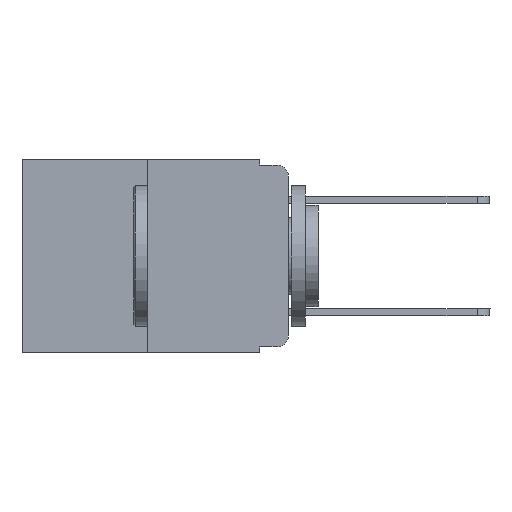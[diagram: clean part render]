
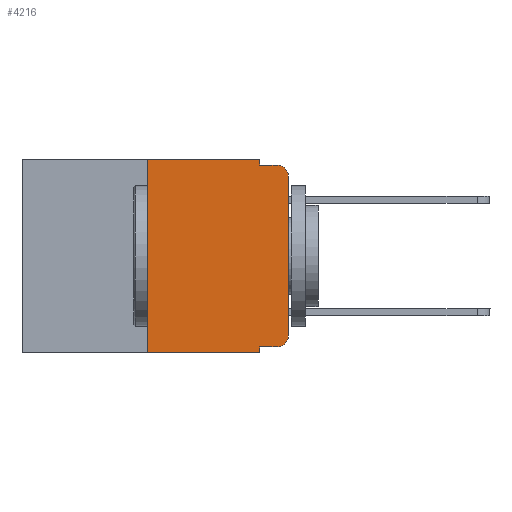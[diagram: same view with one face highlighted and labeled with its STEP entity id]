
A CAD part, left-side view. The second image highlights one B-rep face of the part: STEP entity #4216.
In plain terms, the highlighted planar face has unit normal (-1, 0, 0).
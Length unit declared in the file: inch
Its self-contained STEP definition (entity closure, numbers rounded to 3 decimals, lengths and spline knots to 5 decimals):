
#224 = ORIENTED_EDGE ( 'NONE', *, *, #13883, .T. ) ;
#556 = LINE ( 'NONE', #5082, #10669 ) ;
#725 = VECTOR ( 'NONE', #8430, 39.37008 ) ;
#908 = EDGE_CURVE ( 'NONE', #1152, #7854, #7517, .T. ) ;
#1152 = VERTEX_POINT ( 'NONE', #13057 ) ;
#1325 = DIRECTION ( 'NONE',  ( -1., 0., 0. ) ) ;
#1409 = CARTESIAN_POINT ( 'NONE',  ( 0., 0.02, -0.03 ) ) ;
#1571 = CARTESIAN_POINT ( 'NONE',  ( 0., 0.051, 0. ) ) ;
#1823 = ORIENTED_EDGE ( 'NONE', *, *, #12660, .F. ) ;
#1828 = CARTESIAN_POINT ( 'NONE',  ( 0., 0.051, -0.333 ) ) ;
#2063 = EDGE_CURVE ( 'NONE', #11426, #9541, #12813, .T. ) ;
#2077 = CARTESIAN_POINT ( 'NONE',  ( 0., 0.051, 0. ) ) ;
#2454 = DIRECTION ( 'NONE',  ( 0., 0., -1. ) ) ;
#2556 = VERTEX_POINT ( 'NONE', #7157 ) ;
#2661 = DIRECTION ( 'NONE',  ( 0., -1., 0. ) ) ;
#2737 = CARTESIAN_POINT ( 'NONE',  ( 0., 0.051, -0.333 ) ) ;
#2764 = LINE ( 'NONE', #1571, #7536 ) ;
#2934 = CARTESIAN_POINT ( 'NONE',  ( 0., 0.051, -0.01 ) ) ;
#2997 = LINE ( 'NONE', #7599, #7765 ) ;
#3192 = LINE ( 'NONE', #7786, #13765 ) ;
#3325 = CARTESIAN_POINT ( 'NONE',  ( 0., 0.25, 0. ) ) ;
#3381 = EDGE_CURVE ( 'NONE', #8652, #2556, #13939, .T. ) ;
#3632 = CARTESIAN_POINT ( 'NONE',  ( 0., 0.051, -0.343 ) ) ;
#3684 = CARTESIAN_POINT ( 'NONE',  ( 0., 0.25, -0.343 ) ) ;
#3817 = VECTOR ( 'NONE', #10365, 39.37008 ) ;
#4088 = ORIENTED_EDGE ( 'NONE', *, *, #12027, .F. ) ;
#4192 = CARTESIAN_POINT ( 'NONE',  ( 0., 0., -0.313 ) ) ;
#4216 = ADVANCED_FACE ( 'NONE', ( #6705 ), #11207, .F. ) ;
#4505 = CARTESIAN_POINT ( 'NONE',  ( 0., 0.02, -0.313 ) ) ;
#4731 = AXIS2_PLACEMENT_3D ( 'NONE', #1409, #5857, #4754 ) ;
#4754 = DIRECTION ( 'NONE',  ( 0., 0., -1. ) ) ;
#5082 = CARTESIAN_POINT ( 'NONE',  ( 0., 0.473, 0. ) ) ;
#5104 = VECTOR ( 'NONE', #2661, 39.37008 ) ;
#5243 = AXIS2_PLACEMENT_3D ( 'NONE', #10107, #11272, #5795 ) ;
#5773 = VERTEX_POINT ( 'NONE', #3684 ) ;
#5795 = DIRECTION ( 'NONE',  ( 0., 0., -1. ) ) ;
#5857 = DIRECTION ( 'NONE',  ( -1., 0., 0. ) ) ;
#6705 = FACE_OUTER_BOUND ( 'NONE', #10676, .T. ) ;
#6773 = CARTESIAN_POINT ( 'NONE',  ( 0., 0.02, -0.01 ) ) ;
#6897 = VERTEX_POINT ( 'NONE', #2077 ) ;
#7157 = CARTESIAN_POINT ( 'NONE',  ( 0., 0., -0.03 ) ) ;
#7492 = ORIENTED_EDGE ( 'NONE', *, *, #3381, .T. ) ;
#7517 = LINE ( 'NONE', #2934, #8426 ) ;
#7536 = VECTOR ( 'NONE', #12849, 39.37008 ) ;
#7592 = EDGE_CURVE ( 'NONE', #11675, #6897, #556, .T. ) ;
#7599 = CARTESIAN_POINT ( 'NONE',  ( 0., 0.051, 0. ) ) ;
#7765 = VECTOR ( 'NONE', #13241, 39.37008 ) ;
#7786 = CARTESIAN_POINT ( 'NONE',  ( 0., 0.473, -0.343 ) ) ;
#7854 = VERTEX_POINT ( 'NONE', #6773 ) ;
#8384 = EDGE_CURVE ( 'NONE', #5773, #8442, #3192, .T. ) ;
#8426 = VECTOR ( 'NONE', #14430, 39.37008 ) ;
#8430 = DIRECTION ( 'NONE',  ( 0., 0., 1. ) ) ;
#8442 = VERTEX_POINT ( 'NONE', #3632 ) ;
#8581 = AXIS2_PLACEMENT_3D ( 'NONE', #4505, #1325, #2454 ) ;
#8652 = VERTEX_POINT ( 'NONE', #4192 ) ;
#8832 = ORIENTED_EDGE ( 'NONE', *, *, #9947, .T. ) ;
#8899 = EDGE_CURVE ( 'NONE', #5773, #11675, #12601, .T. ) ;
#9401 = CARTESIAN_POINT ( 'NONE',  ( 0., 0.25, 0. ) ) ;
#9541 = VERTEX_POINT ( 'NONE', #13545 ) ;
#9947 = EDGE_CURVE ( 'NONE', #9541, #8652, #10498, .T. ) ;
#10107 = CARTESIAN_POINT ( 'NONE',  ( 0., 0.473, 0. ) ) ;
#10365 = DIRECTION ( 'NONE',  ( 0., 0., 1. ) ) ;
#10498 = CIRCLE ( 'NONE', #8581, 0.02 ) ;
#10669 = VECTOR ( 'NONE', #13999, 39.37008 ) ;
#10676 = EDGE_LOOP ( 'NONE', ( #7492, #224, #13871, #1823, #10942, #11573, #13231, #4088, #14575, #8832 ) ) ;
#10873 = CIRCLE ( 'NONE', #4731, 0.02 ) ;
#10942 = ORIENTED_EDGE ( 'NONE', *, *, #7592, .F. ) ;
#11207 = PLANE ( 'NONE',  #5243 ) ;
#11272 = DIRECTION ( 'NONE',  ( 1., 0., 0. ) ) ;
#11330 = DIRECTION ( 'NONE',  ( 0., -1., 0. ) ) ;
#11426 = VERTEX_POINT ( 'NONE', #1828 ) ;
#11573 = ORIENTED_EDGE ( 'NONE', *, *, #8899, .F. ) ;
#11675 = VERTEX_POINT ( 'NONE', #3325 ) ;
#12027 = EDGE_CURVE ( 'NONE', #11426, #8442, #2997, .T. ) ;
#12601 = LINE ( 'NONE', #9401, #3817 ) ;
#12660 = EDGE_CURVE ( 'NONE', #6897, #1152, #2764, .T. ) ;
#12813 = LINE ( 'NONE', #2737, #5104 ) ;
#12849 = DIRECTION ( 'NONE',  ( 0., 0., -1. ) ) ;
#12897 = CARTESIAN_POINT ( 'NONE',  ( 0., 0., 0. ) ) ;
#13057 = CARTESIAN_POINT ( 'NONE',  ( 0., 0.051, -0.01 ) ) ;
#13231 = ORIENTED_EDGE ( 'NONE', *, *, #8384, .T. ) ;
#13241 = DIRECTION ( 'NONE',  ( 0., 0., -1. ) ) ;
#13545 = CARTESIAN_POINT ( 'NONE',  ( 0., 0.02, -0.333 ) ) ;
#13765 = VECTOR ( 'NONE', #11330, 39.37008 ) ;
#13871 = ORIENTED_EDGE ( 'NONE', *, *, #908, .F. ) ;
#13883 = EDGE_CURVE ( 'NONE', #2556, #7854, #10873, .T. ) ;
#13939 = LINE ( 'NONE', #12897, #725 ) ;
#13999 = DIRECTION ( 'NONE',  ( 0., -1., 0. ) ) ;
#14430 = DIRECTION ( 'NONE',  ( 0., -1., 0. ) ) ;
#14575 = ORIENTED_EDGE ( 'NONE', *, *, #2063, .T. ) ;
